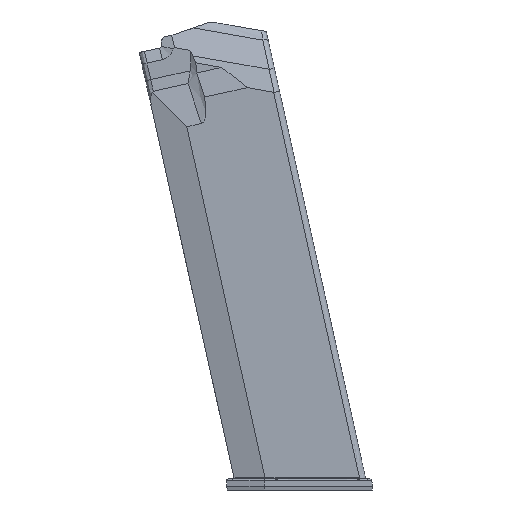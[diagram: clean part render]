
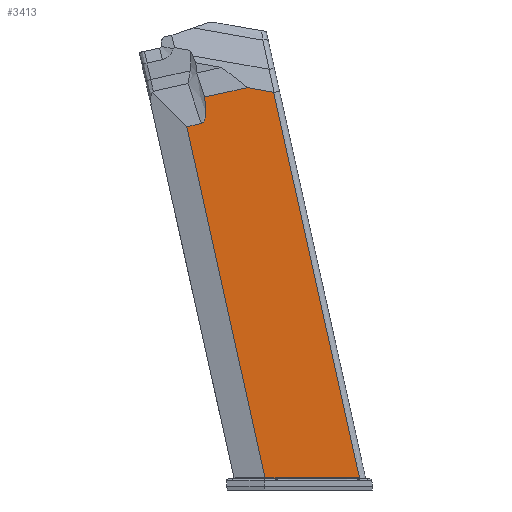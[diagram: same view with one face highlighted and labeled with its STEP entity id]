
A CAD part, left-side view. The second image highlights one B-rep face of the part: STEP entity #3413.
In plain terms, the highlighted planar face has unit normal (-1, 0, 0).
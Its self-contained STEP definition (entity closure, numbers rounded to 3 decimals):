
#188=FACE_OUTER_BOUND('',#385,.T.);
#385=EDGE_LOOP('',(#2474,#2475,#2476,#2477,#2478,#2479,#2480,#2481));
#562=ELLIPSE('',#3628,1.083,0.25);
#657=LINE('',#4459,#913);
#695=LINE('',#5047,#951);
#701=LINE('',#5070,#957);
#756=LINE('',#5411,#1012);
#758=LINE('',#5453,#1014);
#759=LINE('',#5454,#1015);
#913=VECTOR('',#3782,10.002);
#951=VECTOR('',#3868,10.);
#957=VECTOR('',#3880,10.039);
#1012=VECTOR('',#4003,10.04);
#1014=VECTOR('',#4013,10.038);
#1015=VECTOR('',#4014,10.002);
#1206=B_SPLINE_CURVE_WITH_KNOTS('',3,(#5440,#5441,#5442,#5443,#5444,#5445,
#5446,#5447,#5448,#5449,#5450,#5451,#5452),.UNSPECIFIED.,.F.,.F.,(4,3,3,
3,4),(0.433,0.612,0.907,1.091,
1.202),.UNSPECIFIED.);
#1334=VERTEX_POINT('',#4456);
#1335=VERTEX_POINT('',#4458);
#1397=VERTEX_POINT('',#5032);
#1398=VERTEX_POINT('',#5046);
#1404=VERTEX_POINT('',#5069);
#1457=VERTEX_POINT('',#5325);
#1462=VERTEX_POINT('',#5402);
#1465=VERTEX_POINT('',#5439);
#1677=EDGE_CURVE('',#1335,#1334,#657,.T.);
#1754=EDGE_CURVE('',#1398,#1397,#695,.T.);
#1762=EDGE_CURVE('',#1398,#1404,#701,.T.);
#1836=EDGE_CURVE('',#1457,#1334,#562,.T.);
#1847=EDGE_CURVE('',#1462,#1457,#756,.T.);
#1852=EDGE_CURVE('',#1465,#1397,#1206,.F.);
#1853=EDGE_CURVE('',#1335,#1465,#758,.T.);
#1854=EDGE_CURVE('',#1404,#1462,#759,.T.);
#2474=ORIENTED_EDGE('',*,*,#1754,.T.);
#2475=ORIENTED_EDGE('',*,*,#1852,.F.);
#2476=ORIENTED_EDGE('',*,*,#1853,.F.);
#2477=ORIENTED_EDGE('',*,*,#1677,.T.);
#2478=ORIENTED_EDGE('',*,*,#1836,.F.);
#2479=ORIENTED_EDGE('',*,*,#1847,.F.);
#2480=ORIENTED_EDGE('',*,*,#1854,.F.);
#2481=ORIENTED_EDGE('',*,*,#1762,.F.);
#3312=PLANE('',#3640);
#3413=ADVANCED_FACE('',(#188),#3312,.T.);
#3628=AXIS2_PLACEMENT_3D('',#5327,#3983,#3984);
#3640=AXIS2_PLACEMENT_3D('',#5438,#4011,#4012);
#3782=DIRECTION('',(0.,-0.217,-0.976));
#3868=DIRECTION('',(0.,0.976,-0.217));
#3880=DIRECTION('',(0.,-0.985,-0.173));
#3983=DIRECTION('center_axis',(-1.,0.,0.));
#3984=DIRECTION('ref_axis',(0.,-1.,0.));
#4003=DIRECTION('',(0.,1.,0.));
#4011=DIRECTION('center_axis',(-1.,0.,0.));
#4012=DIRECTION('ref_axis',(0.,0.,1.));
#4013=DIRECTION('',(0.,-0.976,0.216));
#4014=DIRECTION('',(0.,-0.217,-0.976));
#4456=CARTESIAN_POINT('',(-10.542,9.511,3.063));
#4458=CARTESIAN_POINT('',(-10.542,29.379,92.322));
#4459=CARTESIAN_POINT('',(-10.542,4.899,-17.657));
#5032=CARTESIAN_POINT('',(-10.542,24.794,99.857));
#5046=CARTESIAN_POINT('',(-10.542,14.048,102.249));
#5047=CARTESIAN_POINT('',(-10.542,15.441,101.939));
#5069=CARTESIAN_POINT('',(-10.542,7.312,101.067));
#5070=CARTESIAN_POINT('',(-10.542,-11.626,97.741));
#5325=CARTESIAN_POINT('',(-10.542,9.51,3.05));
#5327=CARTESIAN_POINT('Origin',(-10.542,10.592,3.05));
#5402=CARTESIAN_POINT('',(-10.542,-14.504,3.05));
#5411=CARTESIAN_POINT('',(-10.542,-9.248,3.05));
#5438=CARTESIAN_POINT('Origin',(-10.542,-19.459,-12.279));
#5439=CARTESIAN_POINT('',(-10.542,25.666,93.142));
#5440=CARTESIAN_POINT('Ctrl Pts',(-10.542,24.794,99.857));
#5441=CARTESIAN_POINT('Ctrl Pts',(-10.542,24.726,99.253));
#5442=CARTESIAN_POINT('Ctrl Pts',(-10.542,24.668,98.644));
#5443=CARTESIAN_POINT('Ctrl Pts',(-10.542,24.628,98.003));
#5444=CARTESIAN_POINT('Ctrl Pts',(-10.542,24.561,96.95));
#5445=CARTESIAN_POINT('Ctrl Pts',(-10.542,24.549,95.875));
#5446=CARTESIAN_POINT('Ctrl Pts',(-10.542,24.665,95.003));
#5447=CARTESIAN_POINT('Ctrl Pts',(-10.542,24.737,94.458));
#5448=CARTESIAN_POINT('Ctrl Pts',(-10.542,24.846,93.987));
#5449=CARTESIAN_POINT('Ctrl Pts',(-10.542,25.076,93.611));
#5450=CARTESIAN_POINT('Ctrl Pts',(-10.542,25.215,93.384));
#5451=CARTESIAN_POINT('Ctrl Pts',(-10.542,25.413,93.198));
#5452=CARTESIAN_POINT('Ctrl Pts',(-10.542,25.666,93.142));
#5453=CARTESIAN_POINT('',(-10.542,20.949,94.184));
#5454=CARTESIAN_POINT('',(-10.542,-17.989,-12.603));
